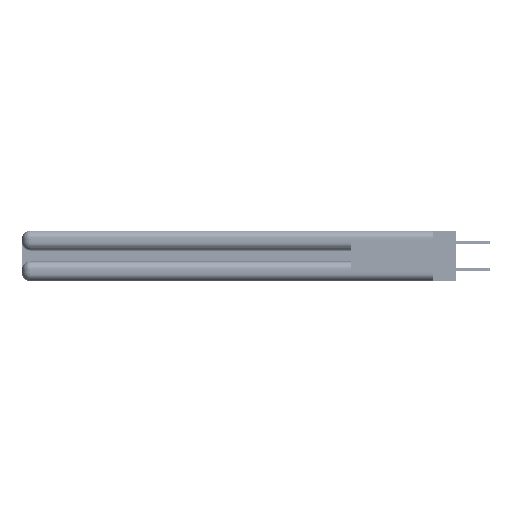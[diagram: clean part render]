
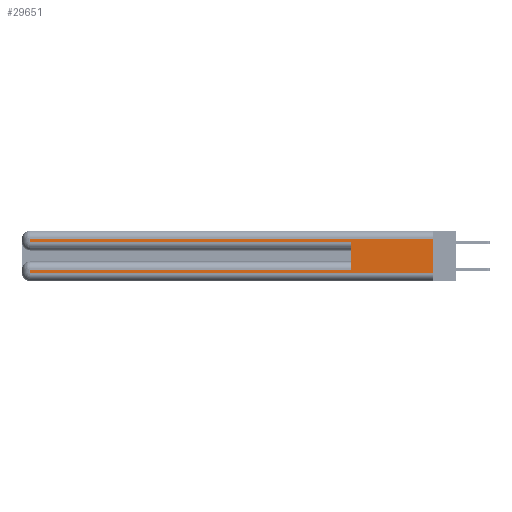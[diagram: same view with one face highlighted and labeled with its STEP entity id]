
A CAD part, left-side view. The second image highlights one B-rep face of the part: STEP entity #29651.
In plain terms, the highlighted planar face has unit normal (-1, 0, 0).
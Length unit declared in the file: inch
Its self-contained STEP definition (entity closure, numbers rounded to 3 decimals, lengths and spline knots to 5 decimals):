
#1772 = DIRECTION ( 'NONE',  ( 1., 0., 0. ) ) ;
#2117 = VECTOR ( 'NONE', #22372, 39.37008 ) ;
#2183 = DIRECTION ( 'NONE',  ( 0., -1., 0. ) ) ;
#3022 = LINE ( 'NONE', #48989, #15332 ) ;
#3476 = CARTESIAN_POINT ( 'NONE',  ( 0., 2.94, 0.37 ) ) ;
#3853 = DIRECTION ( 'NONE',  ( 0., 0., -1. ) ) ;
#3882 = CARTESIAN_POINT ( 'NONE',  ( 0., 2.94, 0.37 ) ) ;
#4578 = VERTEX_POINT ( 'NONE', #22991 ) ;
#4944 = DIRECTION ( 'NONE',  ( 0., 0., -1. ) ) ;
#5116 = DIRECTION ( 'NONE',  ( 0., 0., 1. ) ) ;
#5773 = CARTESIAN_POINT ( 'NONE',  ( 0., 0., 0.37 ) ) ;
#8030 = EDGE_CURVE ( 'NONE', #41084, #8851, #38081, .T. ) ;
#8503 = VECTOR ( 'NONE', #43973, 39.37008 ) ;
#8851 = VERTEX_POINT ( 'NONE', #38263 ) ;
#9425 = ORIENTED_EDGE ( 'NONE', *, *, #26739, .T. ) ;
#10598 = CARTESIAN_POINT ( 'NONE',  ( 0., 0., 0.06 ) ) ;
#11340 = ORIENTED_EDGE ( 'NONE', *, *, #33224, .T. ) ;
#11740 = EDGE_CURVE ( 'NONE', #43452, #4578, #54156, .T. ) ;
#12073 = CARTESIAN_POINT ( 'NONE',  ( 0., 0., 0.31 ) ) ;
#13062 = CARTESIAN_POINT ( 'NONE',  ( 0., 0.6, 0.085 ) ) ;
#15332 = VECTOR ( 'NONE', #5116, 39.37008 ) ;
#18454 = DIRECTION ( 'NONE',  ( 0., 1., 0. ) ) ;
#19354 = AXIS2_PLACEMENT_3D ( 'NONE', #5773, #1772, #39753 ) ;
#19824 = ORIENTED_EDGE ( 'NONE', *, *, #8030, .T. ) ;
#20322 = EDGE_CURVE ( 'NONE', #43452, #41084, #52945, .T. ) ;
#21172 = ORIENTED_EDGE ( 'NONE', *, *, #11740, .F. ) ;
#22372 = DIRECTION ( 'NONE',  ( 0., -1., 0. ) ) ;
#22832 = CARTESIAN_POINT ( 'NONE',  ( 0., 0., 0.085 ) ) ;
#22991 = CARTESIAN_POINT ( 'NONE',  ( 0., 0., 0.06 ) ) ;
#24339 = DIRECTION ( 'NONE',  ( 0., 1., 0. ) ) ;
#25398 = CARTESIAN_POINT ( 'NONE',  ( 0., 0., 0.31 ) ) ;
#26739 = EDGE_CURVE ( 'NONE', #32205, #51450, #41623, .T. ) ;
#26753 = CARTESIAN_POINT ( 'NONE',  ( 0., 0., 0.285 ) ) ;
#26754 = CARTESIAN_POINT ( 'NONE',  ( 0., 0., 0.37 ) ) ;
#29488 = LINE ( 'NONE', #26753, #2117 ) ;
#29651 = ADVANCED_FACE ( 'NONE', ( #40598 ), #45086, .F. ) ;
#30307 = ORIENTED_EDGE ( 'NONE', *, *, #48895, .T. ) ;
#32205 = VERTEX_POINT ( 'NONE', #13062 ) ;
#33224 = EDGE_CURVE ( 'NONE', #35996, #4578, #43444, .T. ) ;
#33244 = VECTOR ( 'NONE', #2183, 39.37008 ) ;
#34351 = EDGE_CURVE ( 'NONE', #32205, #44277, #3022, .T. ) ;
#35803 = EDGE_LOOP ( 'NONE', ( #21172, #39420, #19824, #30307, #53676, #9425, #38155, #11340 ) ) ;
#35996 = VERTEX_POINT ( 'NONE', #49160 ) ;
#36861 = VECTOR ( 'NONE', #18454, 39.37008 ) ;
#38081 = LINE ( 'NONE', #3476, #53716 ) ;
#38155 = ORIENTED_EDGE ( 'NONE', *, *, #46824, .T. ) ;
#38263 = CARTESIAN_POINT ( 'NONE',  ( 0., 2.94, 0.285 ) ) ;
#38538 = LINE ( 'NONE', #3882, #8503 ) ;
#39420 = ORIENTED_EDGE ( 'NONE', *, *, #20322, .T. ) ;
#39540 = CARTESIAN_POINT ( 'NONE',  ( 0., 2.94, 0.085 ) ) ;
#39753 = DIRECTION ( 'NONE',  ( 0., 0., -1. ) ) ;
#40598 = FACE_OUTER_BOUND ( 'NONE', #35803, .T. ) ;
#40986 = CARTESIAN_POINT ( 'NONE',  ( 0., 0.6, 0.285 ) ) ;
#41084 = VERTEX_POINT ( 'NONE', #55722 ) ;
#41623 = LINE ( 'NONE', #22832, #36861 ) ;
#43444 = LINE ( 'NONE', #10598, #33244 ) ;
#43452 = VERTEX_POINT ( 'NONE', #25398 ) ;
#43973 = DIRECTION ( 'NONE',  ( 0., 0., -1. ) ) ;
#44277 = VERTEX_POINT ( 'NONE', #40986 ) ;
#45086 = PLANE ( 'NONE',  #19354 ) ;
#46824 = EDGE_CURVE ( 'NONE', #51450, #35996, #38538, .T. ) ;
#48895 = EDGE_CURVE ( 'NONE', #8851, #44277, #29488, .T. ) ;
#48989 = CARTESIAN_POINT ( 'NONE',  ( 0., 0.6, 0.145 ) ) ;
#49160 = CARTESIAN_POINT ( 'NONE',  ( 0., 2.94, 0.06 ) ) ;
#49350 = VECTOR ( 'NONE', #4944, 39.37008 ) ;
#51450 = VERTEX_POINT ( 'NONE', #39540 ) ;
#52945 = LINE ( 'NONE', #12073, #53595 ) ;
#53595 = VECTOR ( 'NONE', #24339, 39.37008 ) ;
#53676 = ORIENTED_EDGE ( 'NONE', *, *, #34351, .F. ) ;
#53716 = VECTOR ( 'NONE', #3853, 39.37008 ) ;
#54156 = LINE ( 'NONE', #26754, #49350 ) ;
#55722 = CARTESIAN_POINT ( 'NONE',  ( 0., 2.94, 0.31 ) ) ;
